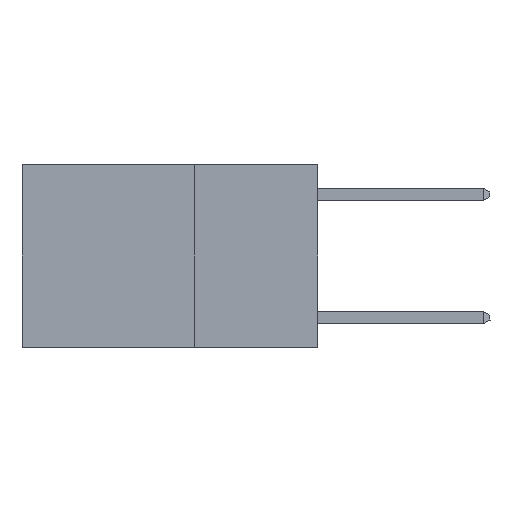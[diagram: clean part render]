
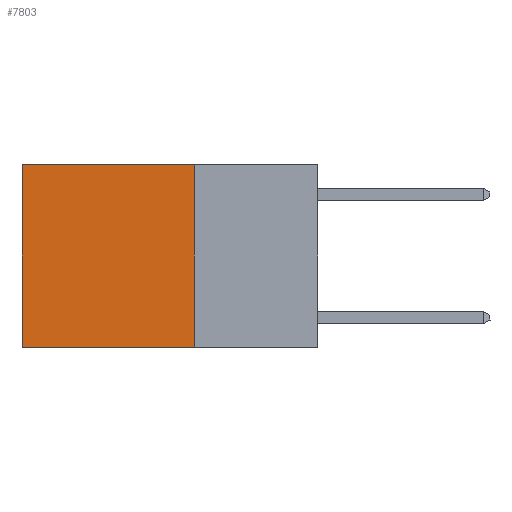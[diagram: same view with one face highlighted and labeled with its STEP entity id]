
A CAD part, left-side view. The second image highlights one B-rep face of the part: STEP entity #7803.
In plain terms, the highlighted planar face has unit normal (-1, 0, 0).
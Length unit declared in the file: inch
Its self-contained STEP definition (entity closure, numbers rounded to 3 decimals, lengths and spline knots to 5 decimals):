
#761 = CARTESIAN_POINT ( 'NONE',  ( 0.2625, 0.6, 0. ) ) ;
#1778 = DIRECTION ( 'NONE',  ( 1., 0., 0. ) ) ;
#1910 = CARTESIAN_POINT ( 'NONE',  ( 0.2625, 0.6, 0. ) ) ;
#2921 = LINE ( 'NONE', #22465, #18922 ) ;
#4941 = EDGE_LOOP ( 'NONE', ( #16445, #13412, #13263, #15277 ) ) ;
#7803 = ADVANCED_FACE ( 'NONE', ( #22992 ), #14385, .F. ) ;
#8372 = DIRECTION ( 'NONE',  ( 0., 0., -1. ) ) ;
#8971 = AXIS2_PLACEMENT_3D ( 'NONE', #20473, #1778, #16461 ) ;
#10238 = CARTESIAN_POINT ( 'NONE',  ( 0.2625, 0.6, -0.37 ) ) ;
#10316 = CARTESIAN_POINT ( 'NONE',  ( 0.2625, 0.25, -0.37 ) ) ;
#12206 = DIRECTION ( 'NONE',  ( 0., 1., 0. ) ) ;
#12506 = CARTESIAN_POINT ( 'NONE',  ( 0.2625, 0.25, -0.37 ) ) ;
#13263 = ORIENTED_EDGE ( 'NONE', *, *, #16071, .F. ) ;
#13412 = ORIENTED_EDGE ( 'NONE', *, *, #20947, .F. ) ;
#14385 = PLANE ( 'NONE',  #8971 ) ;
#14445 = VECTOR ( 'NONE', #22853, 39.37008 ) ;
#14842 = CARTESIAN_POINT ( 'NONE',  ( 0.2625, 0.25, 0. ) ) ;
#14893 = VECTOR ( 'NONE', #15465, 39.37008 ) ;
#15277 = ORIENTED_EDGE ( 'NONE', *, *, #21204, .T. ) ;
#15465 = DIRECTION ( 'NONE',  ( 0., 0., -1. ) ) ;
#16071 = EDGE_CURVE ( 'NONE', #19726, #18011, #18620, .T. ) ;
#16445 = ORIENTED_EDGE ( 'NONE', *, *, #25599, .T. ) ;
#16461 = DIRECTION ( 'NONE',  ( 0., 0., -1. ) ) ;
#18011 = VERTEX_POINT ( 'NONE', #10316 ) ;
#18620 = LINE ( 'NONE', #20793, #24078 ) ;
#18922 = VECTOR ( 'NONE', #12206, 39.37008 ) ;
#19726 = VERTEX_POINT ( 'NONE', #14842 ) ;
#20473 = CARTESIAN_POINT ( 'NONE',  ( 0.2625, 0.25, 0. ) ) ;
#20533 = LINE ( 'NONE', #12506, #14445 ) ;
#20793 = CARTESIAN_POINT ( 'NONE',  ( 0.2625, 0.25, 0. ) ) ;
#20947 = EDGE_CURVE ( 'NONE', #18011, #21921, #20533, .T. ) ;
#21204 = EDGE_CURVE ( 'NONE', #19726, #25295, #2921, .T. ) ;
#21921 = VERTEX_POINT ( 'NONE', #10238 ) ;
#22465 = CARTESIAN_POINT ( 'NONE',  ( 0.2625, 0.25, 0. ) ) ;
#22853 = DIRECTION ( 'NONE',  ( 0., 1., 0. ) ) ;
#22992 = FACE_OUTER_BOUND ( 'NONE', #4941, .T. ) ;
#24078 = VECTOR ( 'NONE', #8372, 39.37008 ) ;
#25295 = VERTEX_POINT ( 'NONE', #1910 ) ;
#25599 = EDGE_CURVE ( 'NONE', #25295, #21921, #25788, .T. ) ;
#25788 = LINE ( 'NONE', #761, #14893 ) ;
